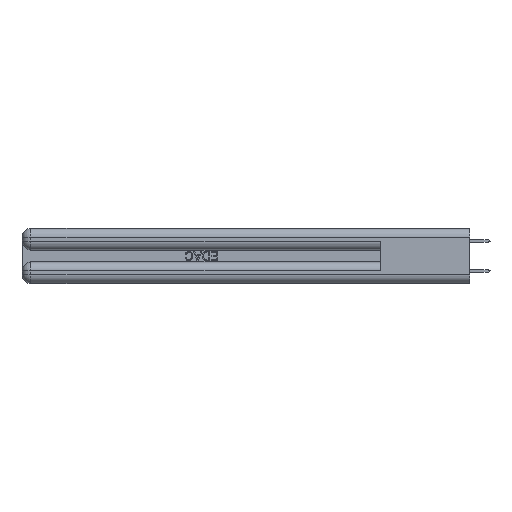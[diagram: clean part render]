
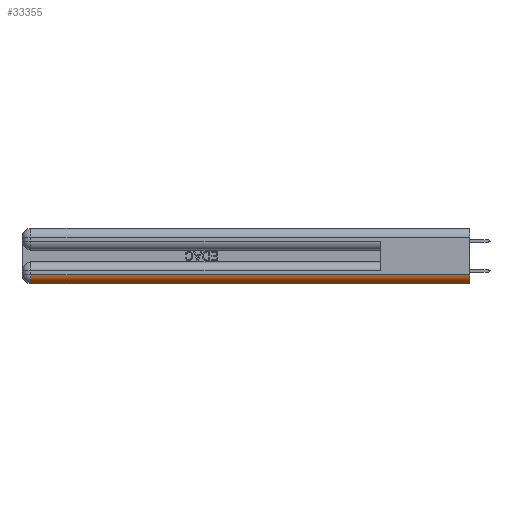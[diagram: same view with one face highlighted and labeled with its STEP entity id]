
A CAD part, left-side view. The second image highlights one B-rep face of the part: STEP entity #33355.
In plain terms, the highlighted cylindrical face has radius 1.524 mm (diameter 3.048 mm), a partial arc.
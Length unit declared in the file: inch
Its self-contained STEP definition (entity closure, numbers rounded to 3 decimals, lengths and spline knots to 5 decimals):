
#4213 = ORIENTED_EDGE ( 'NONE', *, *, #40243, .F. ) ;
#4797 = CARTESIAN_POINT ( 'NONE',  ( 0.06, 0., 0.06 ) ) ;
#5813 = VERTEX_POINT ( 'NONE', #28334 ) ;
#5838 = FACE_OUTER_BOUND ( 'NONE', #23243, .T. ) ;
#6210 = CIRCLE ( 'NONE', #38433, 0.06 ) ;
#6608 = LINE ( 'NONE', #43566, #48299 ) ;
#6622 = VERTEX_POINT ( 'NONE', #16404 ) ;
#6630 = AXIS2_PLACEMENT_3D ( 'NONE', #4797, #20090, #27239 ) ;
#6821 = ORIENTED_EDGE ( 'NONE', *, *, #48245, .F. ) ;
#8346 = DIRECTION ( 'NONE',  ( 0., 1., 0. ) ) ;
#8968 = DIRECTION ( 'NONE',  ( 0., 0., 1. ) ) ;
#9843 = DIRECTION ( 'NONE',  ( 0., -1., 0. ) ) ;
#12059 = CARTESIAN_POINT ( 'NONE',  ( 0.06, 3., 0. ) ) ;
#12273 = DIRECTION ( 'NONE',  ( 0., 1., 0. ) ) ;
#12986 = AXIS2_PLACEMENT_3D ( 'NONE', #45971, #12273, #38844 ) ;
#15186 = VERTEX_POINT ( 'NONE', #31443 ) ;
#16404 = CARTESIAN_POINT ( 'NONE',  ( 0., 0., 0.06 ) ) ;
#19737 = VERTEX_POINT ( 'NONE', #26001 ) ;
#20010 = VECTOR ( 'NONE', #8346, 39.37008 ) ;
#20090 = DIRECTION ( 'NONE',  ( 0., -1., 0. ) ) ;
#23243 = EDGE_LOOP ( 'NONE', ( #29896, #29420, #4213, #6821 ) ) ;
#24256 = DIRECTION ( 'NONE',  ( 0., 1., 0. ) ) ;
#25423 = EDGE_CURVE ( 'NONE', #6622, #19737, #48281, .T. ) ;
#26001 = CARTESIAN_POINT ( 'NONE',  ( 0.06, 0., 0. ) ) ;
#27239 = DIRECTION ( 'NONE',  ( 0., 0., 1. ) ) ;
#28334 = CARTESIAN_POINT ( 'NONE',  ( 0.06, 2.94, 0. ) ) ;
#29420 = ORIENTED_EDGE ( 'NONE', *, *, #33178, .F. ) ;
#29896 = ORIENTED_EDGE ( 'NONE', *, *, #25423, .F. ) ;
#31443 = CARTESIAN_POINT ( 'NONE',  ( 0., 2.94, 0.06 ) ) ;
#33178 = EDGE_CURVE ( 'NONE', #15186, #6622, #6608, .T. ) ;
#33355 = ADVANCED_FACE ( 'NONE', ( #5838 ), #35899, .T. ) ;
#35899 = CYLINDRICAL_SURFACE ( 'NONE', #12986, 0.06 ) ;
#38433 = AXIS2_PLACEMENT_3D ( 'NONE', #47106, #24256, #8968 ) ;
#38844 = DIRECTION ( 'NONE',  ( 0., 0., 1. ) ) ;
#40243 = EDGE_CURVE ( 'NONE', #5813, #15186, #6210, .T. ) ;
#43566 = CARTESIAN_POINT ( 'NONE',  ( 0., 0., 0.06 ) ) ;
#45762 = LINE ( 'NONE', #12059, #20010 ) ;
#45971 = CARTESIAN_POINT ( 'NONE',  ( 0.06, 0., 0.06 ) ) ;
#47106 = CARTESIAN_POINT ( 'NONE',  ( 0.06, 2.94, 0.06 ) ) ;
#48245 = EDGE_CURVE ( 'NONE', #19737, #5813, #45762, .T. ) ;
#48281 = CIRCLE ( 'NONE', #6630, 0.06 ) ;
#48299 = VECTOR ( 'NONE', #9843, 39.37008 ) ;
